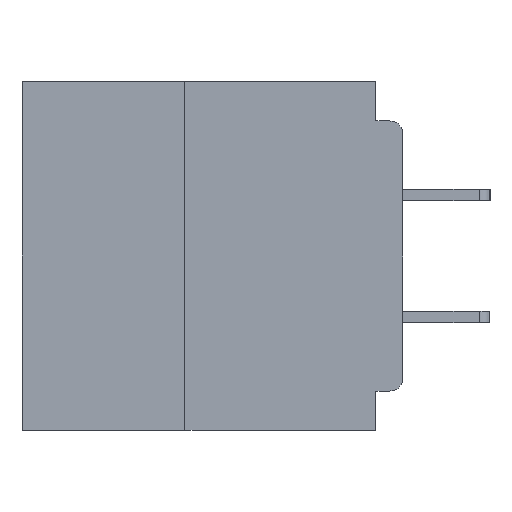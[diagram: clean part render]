
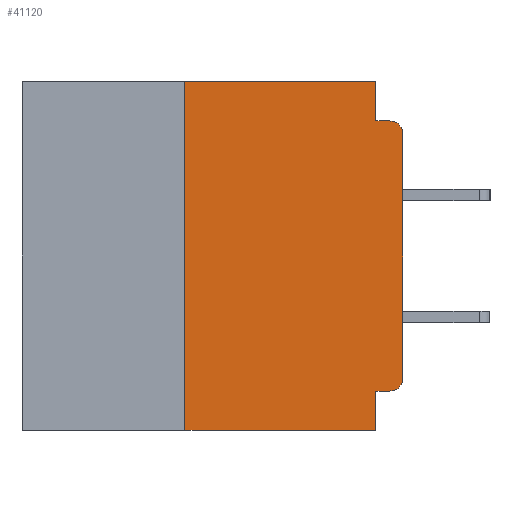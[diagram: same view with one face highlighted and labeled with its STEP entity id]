
A CAD part, left-side view. The second image highlights one B-rep face of the part: STEP entity #41120.
In plain terms, the highlighted planar face has unit normal (-1, 0, 0).
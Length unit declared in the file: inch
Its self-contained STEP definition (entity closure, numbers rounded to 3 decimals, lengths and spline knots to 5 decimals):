
#792 = ORIENTED_EDGE ( 'NONE', *, *, #2102, .T. ) ;
#876 = CARTESIAN_POINT ( 'NONE',  ( 0., 0.031, -0.355 ) ) ;
#1078 = LINE ( 'NONE', #32748, #20888 ) ;
#1098 = DIRECTION ( 'NONE',  ( 0., 0., -1. ) ) ;
#1179 = CARTESIAN_POINT ( 'NONE',  ( 0., 0., -0.045 ) ) ;
#1432 = DIRECTION ( 'NONE',  ( 0., -1., 0. ) ) ;
#1923 = DIRECTION ( 'NONE',  ( 0., -1., 0. ) ) ;
#2007 = CARTESIAN_POINT ( 'NONE',  ( 0., 0.015, -0.355 ) ) ;
#2102 = EDGE_CURVE ( 'NONE', #31657, #29991, #1078, .T. ) ;
#2233 = VECTOR ( 'NONE', #1923, 39.37008 ) ;
#2525 = EDGE_CURVE ( 'NONE', #18742, #42475, #24517, .T. ) ;
#4309 = DIRECTION ( 'NONE',  ( 0., 1., 0. ) ) ;
#5488 = EDGE_CURVE ( 'NONE', #9624, #31657, #7456, .T. ) ;
#5536 = DIRECTION ( 'NONE',  ( 0., 0., -1. ) ) ;
#7456 = CIRCLE ( 'NONE', #21428, 0.015 ) ;
#7669 = LINE ( 'NONE', #37031, #46933 ) ;
#8944 = CARTESIAN_POINT ( 'NONE',  ( 0., 0.031, -0.4 ) ) ;
#9203 = AXIS2_PLACEMENT_3D ( 'NONE', #42756, #50645, #27190 ) ;
#9208 = DIRECTION ( 'NONE',  ( 0., -1., 0. ) ) ;
#9528 = VECTOR ( 'NONE', #1098, 39.37008 ) ;
#9624 = VERTEX_POINT ( 'NONE', #2007 ) ;
#10094 = EDGE_CURVE ( 'NONE', #24915, #42979, #10782, .T. ) ;
#10782 = LINE ( 'NONE', #8944, #9528 ) ;
#13301 = DIRECTION ( 'NONE',  ( -1., 0., 0. ) ) ;
#13722 = ORIENTED_EDGE ( 'NONE', *, *, #2525, .F. ) ;
#15404 = PLANE ( 'NONE',  #9203 ) ;
#15590 = ORIENTED_EDGE ( 'NONE', *, *, #39516, .T. ) ;
#15796 = CARTESIAN_POINT ( 'NONE',  ( 0., 0.031, -0.4 ) ) ;
#16266 = CIRCLE ( 'NONE', #48511, 0.015 ) ;
#17607 = VERTEX_POINT ( 'NONE', #49279 ) ;
#18717 = EDGE_CURVE ( 'NONE', #17607, #38779, #7669, .T. ) ;
#18742 = VERTEX_POINT ( 'NONE', #37209 ) ;
#20888 = VECTOR ( 'NONE', #36683, 39.37008 ) ;
#21428 = AXIS2_PLACEMENT_3D ( 'NONE', #36755, #13301, #40652 ) ;
#21535 = CARTESIAN_POINT ( 'NONE',  ( 0., 0.015, -0.06 ) ) ;
#23388 = VECTOR ( 'NONE', #1432, 39.37008 ) ;
#23447 = DIRECTION ( 'NONE',  ( 0., 0., 1. ) ) ;
#23990 = CARTESIAN_POINT ( 'NONE',  ( 0., 0., -0.355 ) ) ;
#24517 = LINE ( 'NONE', #35274, #46534 ) ;
#24915 = VERTEX_POINT ( 'NONE', #876 ) ;
#25446 = DIRECTION ( 'NONE',  ( 0., 0., -1. ) ) ;
#26234 = CARTESIAN_POINT ( 'NONE',  ( 0., 0.015, -0.045 ) ) ;
#27190 = DIRECTION ( 'NONE',  ( 0., 0., -1. ) ) ;
#29756 = ORIENTED_EDGE ( 'NONE', *, *, #49377, .F. ) ;
#29991 = VERTEX_POINT ( 'NONE', #36601 ) ;
#30144 = FACE_OUTER_BOUND ( 'NONE', #33405, .T. ) ;
#30619 = VECTOR ( 'NONE', #9208, 39.37008 ) ;
#30715 = CARTESIAN_POINT ( 'NONE',  ( 0., 0., -0.34 ) ) ;
#31657 = VERTEX_POINT ( 'NONE', #30715 ) ;
#32748 = CARTESIAN_POINT ( 'NONE',  ( 0., 0., 0. ) ) ;
#33405 = EDGE_LOOP ( 'NONE', ( #792, #15590, #47407, #39608, #29756, #13722, #41255, #43670, #40133, #49235 ) ) ;
#33677 = LINE ( 'NONE', #49022, #2233 ) ;
#35136 = LINE ( 'NONE', #23990, #44254 ) ;
#35274 = CARTESIAN_POINT ( 'NONE',  ( 0., 0.25, -0.4 ) ) ;
#36601 = CARTESIAN_POINT ( 'NONE',  ( 0., 0., -0.06 ) ) ;
#36683 = DIRECTION ( 'NONE',  ( 0., 0., 1. ) ) ;
#36755 = CARTESIAN_POINT ( 'NONE',  ( 0., 0.015, -0.34 ) ) ;
#37031 = CARTESIAN_POINT ( 'NONE',  ( 0., 0.031, 0. ) ) ;
#37209 = CARTESIAN_POINT ( 'NONE',  ( 0., 0.25, -0.4 ) ) ;
#38779 = VERTEX_POINT ( 'NONE', #45562 ) ;
#39516 = EDGE_CURVE ( 'NONE', #29991, #49485, #16266, .T. ) ;
#39608 = ORIENTED_EDGE ( 'NONE', *, *, #18717, .F. ) ;
#40097 = CARTESIAN_POINT ( 'NONE',  ( 0., 0.25, 0. ) ) ;
#40133 = ORIENTED_EDGE ( 'NONE', *, *, #40571, .F. ) ;
#40571 = EDGE_CURVE ( 'NONE', #9624, #24915, #35136, .T. ) ;
#40652 = DIRECTION ( 'NONE',  ( 0., 0., -1. ) ) ;
#41005 = LINE ( 'NONE', #1179, #30619 ) ;
#41120 = ADVANCED_FACE ( 'NONE', ( #30144 ), #15404, .F. ) ;
#41255 = ORIENTED_EDGE ( 'NONE', *, *, #48063, .T. ) ;
#42475 = VERTEX_POINT ( 'NONE', #40097 ) ;
#42756 = CARTESIAN_POINT ( 'NONE',  ( 0., 0.437, 0. ) ) ;
#42979 = VERTEX_POINT ( 'NONE', #15796 ) ;
#43670 = ORIENTED_EDGE ( 'NONE', *, *, #10094, .F. ) ;
#44175 = LINE ( 'NONE', #44540, #23388 ) ;
#44254 = VECTOR ( 'NONE', #4309, 39.37008 ) ;
#44540 = CARTESIAN_POINT ( 'NONE',  ( 0., 0.437, -0.4 ) ) ;
#45562 = CARTESIAN_POINT ( 'NONE',  ( 0., 0.031, -0.045 ) ) ;
#46534 = VECTOR ( 'NONE', #23447, 39.37008 ) ;
#46933 = VECTOR ( 'NONE', #5536, 39.37008 ) ;
#47407 = ORIENTED_EDGE ( 'NONE', *, *, #49890, .F. ) ;
#48063 = EDGE_CURVE ( 'NONE', #18742, #42979, #44175, .T. ) ;
#48511 = AXIS2_PLACEMENT_3D ( 'NONE', #21535, #48904, #25446 ) ;
#48904 = DIRECTION ( 'NONE',  ( -1., 0., 0. ) ) ;
#49022 = CARTESIAN_POINT ( 'NONE',  ( 0., 0.437, 0. ) ) ;
#49235 = ORIENTED_EDGE ( 'NONE', *, *, #5488, .T. ) ;
#49279 = CARTESIAN_POINT ( 'NONE',  ( 0., 0.031, 0. ) ) ;
#49377 = EDGE_CURVE ( 'NONE', #42475, #17607, #33677, .T. ) ;
#49485 = VERTEX_POINT ( 'NONE', #26234 ) ;
#49890 = EDGE_CURVE ( 'NONE', #38779, #49485, #41005, .T. ) ;
#50645 = DIRECTION ( 'NONE',  ( 1., 0., 0. ) ) ;
